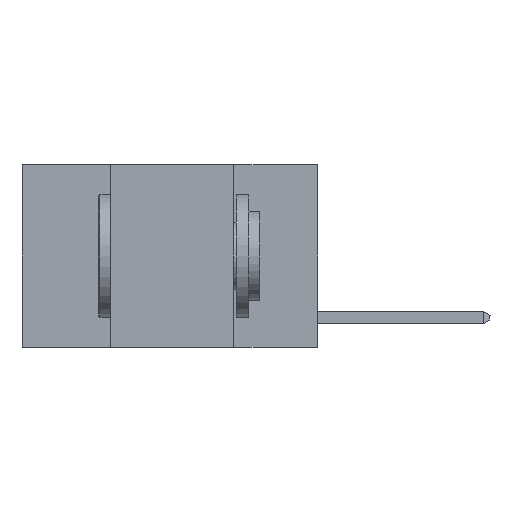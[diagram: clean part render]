
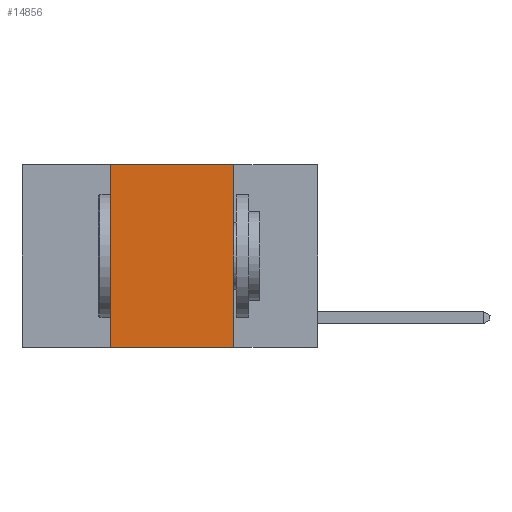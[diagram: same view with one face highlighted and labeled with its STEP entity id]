
A CAD part, left-side view. The second image highlights one B-rep face of the part: STEP entity #14856.
In plain terms, the highlighted planar face has unit normal (-1, 0, 0).
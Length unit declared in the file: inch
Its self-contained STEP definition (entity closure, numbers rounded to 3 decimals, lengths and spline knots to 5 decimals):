
#164 = LINE ( 'NONE', #4129, #2780 ) ;
#234 = EDGE_CURVE ( 'NONE', #17352, #15787, #164, .T. ) ;
#273 = ORIENTED_EDGE ( 'NONE', *, *, #17318, .F. ) ;
#461 = DIRECTION ( 'NONE',  ( 0., 0., -1. ) ) ;
#803 = VERTEX_POINT ( 'NONE', #7529 ) ;
#932 = DIRECTION ( 'NONE',  ( 1., 0., 0. ) ) ;
#936 = AXIS2_PLACEMENT_3D ( 'NONE', #13440, #932, #17734 ) ;
#2780 = VECTOR ( 'NONE', #8480, 39.37008 ) ;
#2993 = VERTEX_POINT ( 'NONE', #9261 ) ;
#3867 = FACE_OUTER_BOUND ( 'NONE', #7363, .T. ) ;
#4129 = CARTESIAN_POINT ( 'NONE',  ( 0., 0.6, 0. ) ) ;
#4135 = VECTOR ( 'NONE', #7796, 39.37008 ) ;
#7363 = EDGE_LOOP ( 'NONE', ( #11262, #14149, #273, #11674 ) ) ;
#7529 = CARTESIAN_POINT ( 'NONE',  ( 0., 0.42, -0.37 ) ) ;
#7796 = DIRECTION ( 'NONE',  ( 0., -1., 0. ) ) ;
#8358 = LINE ( 'NONE', #15381, #9785 ) ;
#8480 = DIRECTION ( 'NONE',  ( 0., -1., 0. ) ) ;
#9261 = CARTESIAN_POINT ( 'NONE',  ( 0., 0.17, -0.37 ) ) ;
#9785 = VECTOR ( 'NONE', #13921, 39.37008 ) ;
#10334 = CARTESIAN_POINT ( 'NONE',  ( 0., 0.17, 0. ) ) ;
#10537 = LINE ( 'NONE', #16128, #4135 ) ;
#11262 = ORIENTED_EDGE ( 'NONE', *, *, #14727, .F. ) ;
#11674 = ORIENTED_EDGE ( 'NONE', *, *, #14491, .T. ) ;
#13440 = CARTESIAN_POINT ( 'NONE',  ( 0., 0.6, 0. ) ) ;
#13921 = DIRECTION ( 'NONE',  ( 0., 0., 1. ) ) ;
#14096 = CARTESIAN_POINT ( 'NONE',  ( 0., 0.42, 0. ) ) ;
#14149 = ORIENTED_EDGE ( 'NONE', *, *, #234, .F. ) ;
#14243 = LINE ( 'NONE', #10334, #15515 ) ;
#14491 = EDGE_CURVE ( 'NONE', #803, #2993, #10537, .T. ) ;
#14727 = EDGE_CURVE ( 'NONE', #15787, #2993, #14243, .T. ) ;
#14856 = ADVANCED_FACE ( 'NONE', ( #3867 ), #17822, .F. ) ;
#15381 = CARTESIAN_POINT ( 'NONE',  ( 0., 0.42, 0. ) ) ;
#15515 = VECTOR ( 'NONE', #461, 39.37008 ) ;
#15787 = VERTEX_POINT ( 'NONE', #16324 ) ;
#16128 = CARTESIAN_POINT ( 'NONE',  ( 0., 0.6, -0.37 ) ) ;
#16324 = CARTESIAN_POINT ( 'NONE',  ( 0., 0.17, 0. ) ) ;
#17318 = EDGE_CURVE ( 'NONE', #803, #17352, #8358, .T. ) ;
#17352 = VERTEX_POINT ( 'NONE', #14096 ) ;
#17734 = DIRECTION ( 'NONE',  ( 0., 0., -1. ) ) ;
#17822 = PLANE ( 'NONE',  #936 ) ;
